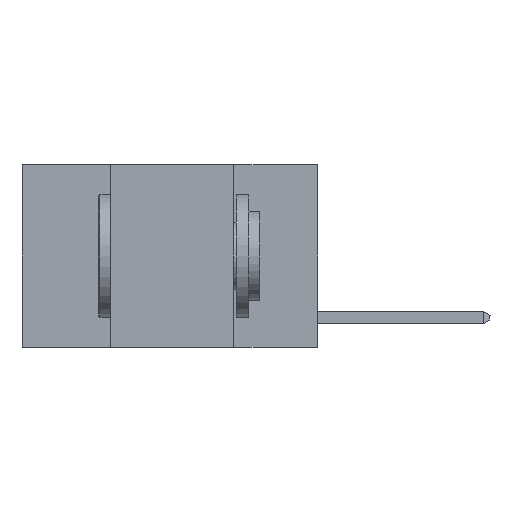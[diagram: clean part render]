
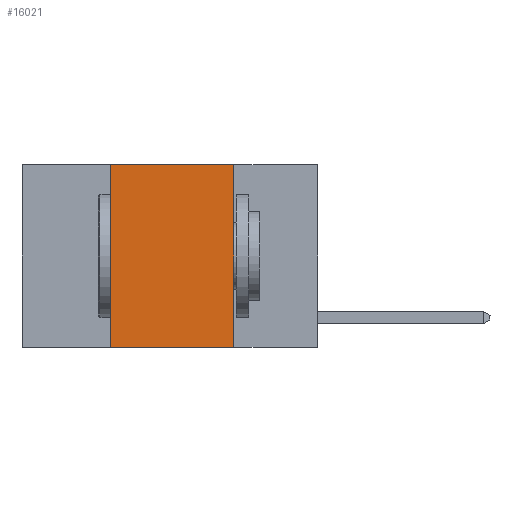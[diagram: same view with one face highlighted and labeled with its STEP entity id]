
A CAD part, left-side view. The second image highlights one B-rep face of the part: STEP entity #16021.
In plain terms, the highlighted planar face has unit normal (-1, 0, 0).
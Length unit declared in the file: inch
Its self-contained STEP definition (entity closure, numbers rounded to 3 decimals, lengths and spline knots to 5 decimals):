
#451 = ORIENTED_EDGE ( 'NONE', *, *, #16351, .F. ) ;
#612 = CARTESIAN_POINT ( 'NONE',  ( 0., 0.17, 0. ) ) ;
#703 = DIRECTION ( 'NONE',  ( 0., 0., -1. ) ) ;
#996 = LINE ( 'NONE', #12178, #5650 ) ;
#1339 = DIRECTION ( 'NONE',  ( 0., -1., 0. ) ) ;
#1993 = CARTESIAN_POINT ( 'NONE',  ( 0., 0.17, -0.37 ) ) ;
#2286 = CARTESIAN_POINT ( 'NONE',  ( 0., 0.6, 0. ) ) ;
#3757 = LINE ( 'NONE', #9774, #13586 ) ;
#4583 = VERTEX_POINT ( 'NONE', #7406 ) ;
#4980 = CARTESIAN_POINT ( 'NONE',  ( 0., 0.6, -0.37 ) ) ;
#5650 = VECTOR ( 'NONE', #9662, 39.37008 ) ;
#5793 = LINE ( 'NONE', #2286, #14832 ) ;
#6966 = VECTOR ( 'NONE', #1339, 39.37008 ) ;
#7406 = CARTESIAN_POINT ( 'NONE',  ( 0., 0.42, -0.37 ) ) ;
#7477 = VERTEX_POINT ( 'NONE', #11683 ) ;
#7784 = ORIENTED_EDGE ( 'NONE', *, *, #11594, .T. ) ;
#8279 = ORIENTED_EDGE ( 'NONE', *, *, #15614, .F. ) ;
#8405 = CARTESIAN_POINT ( 'NONE',  ( 0., 0.6, 0. ) ) ;
#8725 = EDGE_CURVE ( 'NONE', #4583, #7477, #996, .T. ) ;
#9465 = DIRECTION ( 'NONE',  ( 1., 0., 0. ) ) ;
#9605 = AXIS2_PLACEMENT_3D ( 'NONE', #8405, #9465, #703 ) ;
#9662 = DIRECTION ( 'NONE',  ( 0., 0., 1. ) ) ;
#9774 = CARTESIAN_POINT ( 'NONE',  ( 0., 0.17, 0. ) ) ;
#9799 = EDGE_LOOP ( 'NONE', ( #451, #8279, #9943, #7784 ) ) ;
#9943 = ORIENTED_EDGE ( 'NONE', *, *, #8725, .F. ) ;
#11022 = DIRECTION ( 'NONE',  ( 0., 0., -1. ) ) ;
#11594 = EDGE_CURVE ( 'NONE', #4583, #15485, #15401, .T. ) ;
#11683 = CARTESIAN_POINT ( 'NONE',  ( 0., 0.42, 0. ) ) ;
#12178 = CARTESIAN_POINT ( 'NONE',  ( 0., 0.42, 0. ) ) ;
#12553 = DIRECTION ( 'NONE',  ( 0., -1., 0. ) ) ;
#13586 = VECTOR ( 'NONE', #11022, 39.37008 ) ;
#14832 = VECTOR ( 'NONE', #12553, 39.37008 ) ;
#15401 = LINE ( 'NONE', #4980, #6966 ) ;
#15485 = VERTEX_POINT ( 'NONE', #1993 ) ;
#15614 = EDGE_CURVE ( 'NONE', #7477, #16407, #5793, .T. ) ;
#16021 = ADVANCED_FACE ( 'NONE', ( #16642 ), #16118, .F. ) ;
#16118 = PLANE ( 'NONE',  #9605 ) ;
#16351 = EDGE_CURVE ( 'NONE', #16407, #15485, #3757, .T. ) ;
#16407 = VERTEX_POINT ( 'NONE', #612 ) ;
#16642 = FACE_OUTER_BOUND ( 'NONE', #9799, .T. ) ;
